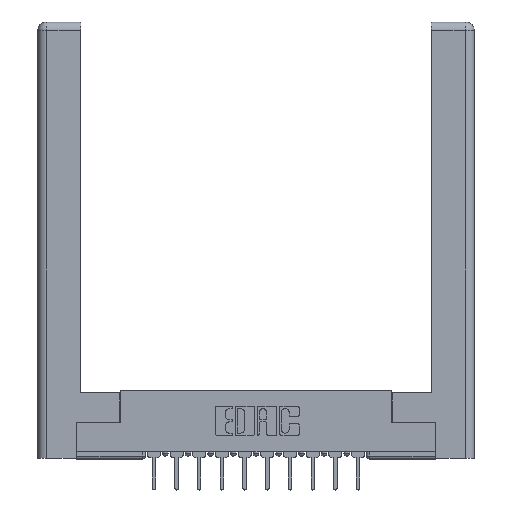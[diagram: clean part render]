
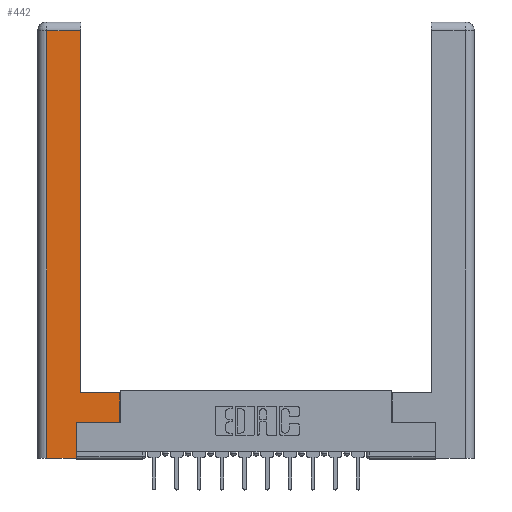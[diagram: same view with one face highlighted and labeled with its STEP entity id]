
A CAD part, top view. The second image highlights one B-rep face of the part: STEP entity #442.
In plain terms, the highlighted planar face has unit normal (0, 0, 1).
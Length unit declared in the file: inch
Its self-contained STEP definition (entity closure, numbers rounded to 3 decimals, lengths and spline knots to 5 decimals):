
#13 = EDGE_CURVE ( 'NONE', #2547, #37, #3002, .T. ) ;
#17 = VECTOR ( 'NONE', #8317, 39.37008 ) ;
#37 = VERTEX_POINT ( 'NONE', #10693 ) ;
#298 = DIRECTION ( 'NONE',  ( 0., 0., -1. ) ) ;
#442 = ADVANCED_FACE ( 'NONE', ( #948 ), #11187, .F. ) ;
#504 = EDGE_CURVE ( 'NONE', #6853, #1181, #7649, .T. ) ;
#554 = DIRECTION ( 'NONE',  ( -1., 0., 0. ) ) ;
#810 = VECTOR ( 'NONE', #8750, 39.37008 ) ;
#948 = FACE_OUTER_BOUND ( 'NONE', #3064, .T. ) ;
#1049 = ORIENTED_EDGE ( 'NONE', *, *, #2259, .T. ) ;
#1181 = VERTEX_POINT ( 'NONE', #4574 ) ;
#1684 = DIRECTION ( 'NONE',  ( 0., 1., 0. ) ) ;
#1757 = VERTEX_POINT ( 'NONE', #14665 ) ;
#1967 = CARTESIAN_POINT ( 'NONE',  ( 0.295, 0.45, 0. ) ) ;
#1973 = CARTESIAN_POINT ( 'NONE',  ( 0.0615, 0., 0. ) ) ;
#2259 = EDGE_CURVE ( 'NONE', #11904, #2547, #2556, .T. ) ;
#2309 = CARTESIAN_POINT ( 'NONE',  ( 0.265, 0., 0. ) ) ;
#2513 = DIRECTION ( 'NONE',  ( 0., 1., 0. ) ) ;
#2547 = VERTEX_POINT ( 'NONE', #6833 ) ;
#2556 = LINE ( 'NONE', #12260, #10814 ) ;
#3002 = LINE ( 'NONE', #4372, #5426 ) ;
#3003 = VERTEX_POINT ( 'NONE', #1973 ) ;
#3064 = EDGE_LOOP ( 'NONE', ( #1049, #12490, #13998, #3326, #11389, #3470, #8248, #3840 ) ) ;
#3251 = LINE ( 'NONE', #10570, #13886 ) ;
#3282 = CARTESIAN_POINT ( 'NONE',  ( 0.565, 0.245, 0. ) ) ;
#3326 = ORIENTED_EDGE ( 'NONE', *, *, #10651, .T. ) ;
#3470 = ORIENTED_EDGE ( 'NONE', *, *, #14388, .T. ) ;
#3506 = LINE ( 'NONE', #3282, #8001 ) ;
#3840 = ORIENTED_EDGE ( 'NONE', *, *, #14927, .T. ) ;
#3871 = VERTEX_POINT ( 'NONE', #6760 ) ;
#4008 = CARTESIAN_POINT ( 'NONE',  ( 0., 0., 0. ) ) ;
#4372 = CARTESIAN_POINT ( 'NONE',  ( 0.0615, 2.94, 0. ) ) ;
#4492 = DIRECTION ( 'NONE',  ( 1., 0., 0. ) ) ;
#4574 = CARTESIAN_POINT ( 'NONE',  ( 0.265, 0.245, 0. ) ) ;
#5426 = VECTOR ( 'NONE', #8013, 39.37008 ) ;
#5613 = VECTOR ( 'NONE', #2513, 39.37008 ) ;
#6516 = CARTESIAN_POINT ( 'NONE',  ( 0.295, 0.45, 0. ) ) ;
#6760 = CARTESIAN_POINT ( 'NONE',  ( 0.565, 0.245, 0. ) ) ;
#6833 = CARTESIAN_POINT ( 'NONE',  ( 0.295, 2.94, 0. ) ) ;
#6853 = VERTEX_POINT ( 'NONE', #2309 ) ;
#7338 = AXIS2_PLACEMENT_3D ( 'NONE', #4008, #298, #14637 ) ;
#7649 = LINE ( 'NONE', #9694, #5613 ) ;
#8001 = VECTOR ( 'NONE', #4492, 39.37008 ) ;
#8013 = DIRECTION ( 'NONE',  ( -1., 0., 0. ) ) ;
#8248 = ORIENTED_EDGE ( 'NONE', *, *, #10237, .T. ) ;
#8317 = DIRECTION ( 'NONE',  ( 1., 0., 0. ) ) ;
#8602 = CARTESIAN_POINT ( 'NONE',  ( 0.565, 0.45, 0. ) ) ;
#8750 = DIRECTION ( 'NONE',  ( 0., 1., 0. ) ) ;
#9391 = LINE ( 'NONE', #8602, #810 ) ;
#9501 = EDGE_CURVE ( 'NONE', #37, #3003, #3251, .T. ) ;
#9694 = CARTESIAN_POINT ( 'NONE',  ( 0.265, 0.245, 0. ) ) ;
#10237 = EDGE_CURVE ( 'NONE', #3871, #1757, #9391, .T. ) ;
#10570 = CARTESIAN_POINT ( 'NONE',  ( 0.0615, 0., 0. ) ) ;
#10651 = EDGE_CURVE ( 'NONE', #3003, #6853, #14383, .T. ) ;
#10693 = CARTESIAN_POINT ( 'NONE',  ( 0.0615, 2.94, 0. ) ) ;
#10814 = VECTOR ( 'NONE', #1684, 39.37008 ) ;
#11187 = PLANE ( 'NONE',  #7338 ) ;
#11389 = ORIENTED_EDGE ( 'NONE', *, *, #504, .T. ) ;
#11904 = VERTEX_POINT ( 'NONE', #1967 ) ;
#12260 = CARTESIAN_POINT ( 'NONE',  ( 0.295, 3., 0. ) ) ;
#12490 = ORIENTED_EDGE ( 'NONE', *, *, #13, .T. ) ;
#13886 = VECTOR ( 'NONE', #15173, 39.37008 ) ;
#13998 = ORIENTED_EDGE ( 'NONE', *, *, #9501, .T. ) ;
#14302 = VECTOR ( 'NONE', #554, 39.37008 ) ;
#14383 = LINE ( 'NONE', #15399, #17 ) ;
#14388 = EDGE_CURVE ( 'NONE', #1181, #3871, #3506, .T. ) ;
#14493 = LINE ( 'NONE', #6516, #14302 ) ;
#14637 = DIRECTION ( 'NONE',  ( -1., 0., 0. ) ) ;
#14665 = CARTESIAN_POINT ( 'NONE',  ( 0.565, 0.45, 0. ) ) ;
#14927 = EDGE_CURVE ( 'NONE', #1757, #11904, #14493, .T. ) ;
#15173 = DIRECTION ( 'NONE',  ( 0., -1., 0. ) ) ;
#15399 = CARTESIAN_POINT ( 'NONE',  ( 0.265, 0., 0. ) ) ;
